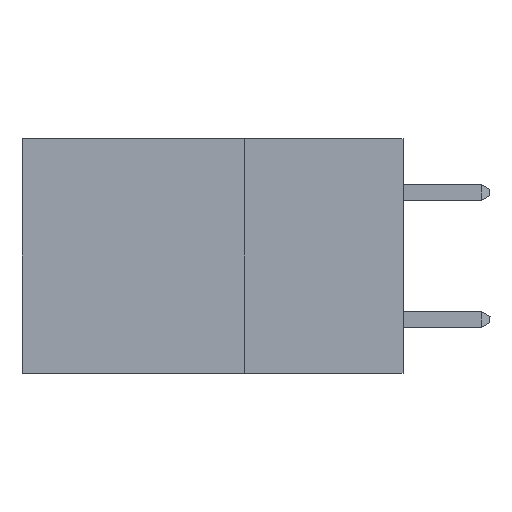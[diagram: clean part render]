
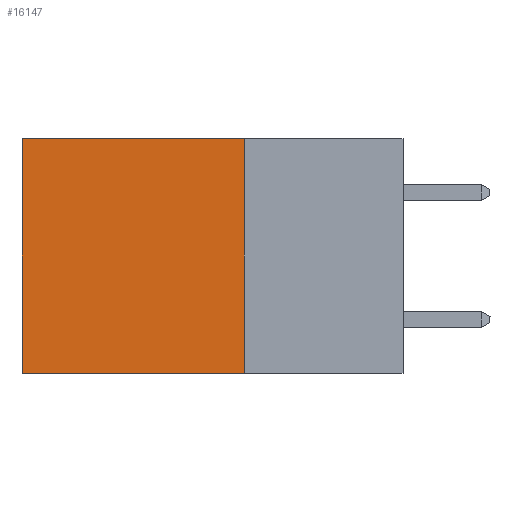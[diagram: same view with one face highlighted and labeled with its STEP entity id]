
A CAD part, left-side view. The second image highlights one B-rep face of the part: STEP entity #16147.
In plain terms, the highlighted planar face has unit normal (-1, 0, 0).
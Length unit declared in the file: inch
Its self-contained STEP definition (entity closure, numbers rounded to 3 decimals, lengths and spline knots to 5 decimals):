
#488 = DIRECTION ( 'NONE',  ( 1., 0., 0. ) ) ;
#2962 = VECTOR ( 'NONE', #42444, 39.37008 ) ;
#3372 = DIRECTION ( 'NONE',  ( 0., 0., -1. ) ) ;
#3558 = CARTESIAN_POINT ( 'NONE',  ( 0.2875, 0.25, 0. ) ) ;
#6311 = ORIENTED_EDGE ( 'NONE', *, *, #17614, .T. ) ;
#7386 = DIRECTION ( 'NONE',  ( 0., 0., -1. ) ) ;
#11086 = EDGE_LOOP ( 'NONE', ( #27037, #22807, #31080, #6311 ) ) ;
#11305 = FACE_OUTER_BOUND ( 'NONE', #11086, .T. ) ;
#13422 = LINE ( 'NONE', #21249, #20190 ) ;
#14899 = CARTESIAN_POINT ( 'NONE',  ( 0.2875, 0.25, 0. ) ) ;
#16147 = ADVANCED_FACE ( 'NONE', ( #11305 ), #41683, .F. ) ;
#17614 = EDGE_CURVE ( 'NONE', #18555, #37393, #13422, .T. ) ;
#18555 = VERTEX_POINT ( 'NONE', #3558 ) ;
#20190 = VECTOR ( 'NONE', #27139, 39.37008 ) ;
#21249 = CARTESIAN_POINT ( 'NONE',  ( 0.2875, 0.25, 0. ) ) ;
#21607 = VERTEX_POINT ( 'NONE', #36901 ) ;
#22807 = ORIENTED_EDGE ( 'NONE', *, *, #39166, .F. ) ;
#25159 = CARTESIAN_POINT ( 'NONE',  ( 0.2875, 0.6, 0. ) ) ;
#26733 = AXIS2_PLACEMENT_3D ( 'NONE', #14899, #488, #38083 ) ;
#27037 = ORIENTED_EDGE ( 'NONE', *, *, #28989, .T. ) ;
#27139 = DIRECTION ( 'NONE',  ( 0., 1., 0. ) ) ;
#27857 = CARTESIAN_POINT ( 'NONE',  ( 0.2875, 0.6, 0. ) ) ;
#28496 = CARTESIAN_POINT ( 'NONE',  ( 0.2875, 0.25, -0.37 ) ) ;
#28989 = EDGE_CURVE ( 'NONE', #37393, #41488, #34627, .T. ) ;
#29637 = VECTOR ( 'NONE', #3372, 39.37008 ) ;
#30434 = CARTESIAN_POINT ( 'NONE',  ( 0.2875, 0.6, -0.37 ) ) ;
#31080 = ORIENTED_EDGE ( 'NONE', *, *, #40318, .F. ) ;
#33118 = VECTOR ( 'NONE', #7386, 39.37008 ) ;
#34627 = LINE ( 'NONE', #25159, #33118 ) ;
#36707 = LINE ( 'NONE', #44348, #29637 ) ;
#36901 = CARTESIAN_POINT ( 'NONE',  ( 0.2875, 0.25, -0.37 ) ) ;
#37393 = VERTEX_POINT ( 'NONE', #27857 ) ;
#38083 = DIRECTION ( 'NONE',  ( 0., 0., -1. ) ) ;
#38619 = LINE ( 'NONE', #28496, #2962 ) ;
#39166 = EDGE_CURVE ( 'NONE', #21607, #41488, #38619, .T. ) ;
#40318 = EDGE_CURVE ( 'NONE', #18555, #21607, #36707, .T. ) ;
#41488 = VERTEX_POINT ( 'NONE', #30434 ) ;
#41683 = PLANE ( 'NONE',  #26733 ) ;
#42444 = DIRECTION ( 'NONE',  ( 0., 1., 0. ) ) ;
#44348 = CARTESIAN_POINT ( 'NONE',  ( 0.2875, 0.25, 0. ) ) ;
